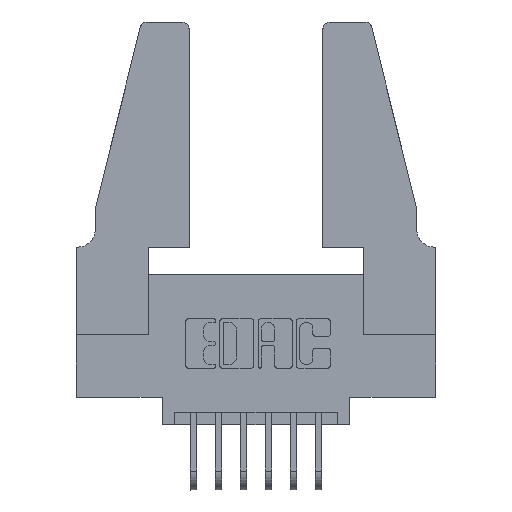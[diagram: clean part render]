
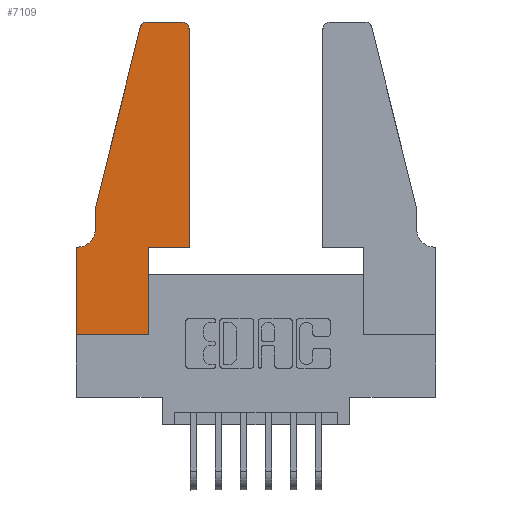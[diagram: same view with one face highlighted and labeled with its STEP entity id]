
A CAD part, top view. The second image highlights one B-rep face of the part: STEP entity #7109.
In plain terms, the highlighted planar face has unit normal (0, 0, 1).
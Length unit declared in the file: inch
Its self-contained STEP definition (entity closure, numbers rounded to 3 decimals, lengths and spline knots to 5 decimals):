
#90 = VECTOR ( 'NONE', #6976, 39.37008 ) ;
#445 = CARTESIAN_POINT ( 'NONE',  ( 0.25487, 1.22718, 0.37 ) ) ;
#467 = CIRCLE ( 'NONE', #1013, 0.03 ) ;
#564 = LINE ( 'NONE', #9493, #90 ) ;
#575 = PLANE ( 'NONE',  #3090 ) ;
#854 = CARTESIAN_POINT ( 'NONE',  ( 0.2605, 1.25, 0.37 ) ) ;
#901 = CIRCLE ( 'NONE', #8744, 0.03 ) ;
#1013 = AXIS2_PLACEMENT_3D ( 'NONE', #11137, #6403, #11711 ) ;
#1124 = CARTESIAN_POINT ( 'NONE',  ( 0.0055, 0.35, 0.37 ) ) ;
#1144 = VECTOR ( 'NONE', #3939, 39.37008 ) ;
#1252 = DIRECTION ( 'NONE',  ( 1., 0., 0. ) ) ;
#1342 = VERTEX_POINT ( 'NONE', #8738 ) ;
#1375 = LINE ( 'NONE', #10201, #1144 ) ;
#1415 = CARTESIAN_POINT ( 'NONE',  ( 0.0755, 0.5, 0.37 ) ) ;
#1596 = CARTESIAN_POINT ( 'NONE',  ( 0.4505, 0.35, 0.37 ) ) ;
#1606 = CARTESIAN_POINT ( 'NONE',  ( 0.4505, 0.35, 0.37 ) ) ;
#1700 = VECTOR ( 'NONE', #6832, 39.37008 ) ;
#1903 = LINE ( 'NONE', #1606, #1700 ) ;
#2016 = CIRCLE ( 'NONE', #2622, 0.07 ) ;
#2067 = EDGE_CURVE ( 'NONE', #8220, #10209, #5675, .T. ) ;
#2543 = VERTEX_POINT ( 'NONE', #445 ) ;
#2622 = AXIS2_PLACEMENT_3D ( 'NONE', #9012, #3261, #9797 ) ;
#3036 = VERTEX_POINT ( 'NONE', #10850 ) ;
#3090 = AXIS2_PLACEMENT_3D ( 'NONE', #6055, #11513, #7043 ) ;
#3141 = DIRECTION ( 'NONE',  ( -1., 0., 0. ) ) ;
#3221 = EDGE_CURVE ( 'NONE', #1342, #3036, #5656, .T. ) ;
#3261 = DIRECTION ( 'NONE',  ( 0., 0., -1. ) ) ;
#3382 = VERTEX_POINT ( 'NONE', #11277 ) ;
#3421 = VECTOR ( 'NONE', #10020, 39.37008 ) ;
#3434 = LINE ( 'NONE', #9252, #3421 ) ;
#3480 = EDGE_CURVE ( 'NONE', #3382, #8220, #1903, .T. ) ;
#3519 = EDGE_CURVE ( 'NONE', #4197, #8986, #1375, .T. ) ;
#3616 = ORIENTED_EDGE ( 'NONE', *, *, #3221, .T. ) ;
#3647 = ORIENTED_EDGE ( 'NONE', *, *, #9417, .T. ) ;
#3939 = DIRECTION ( 'NONE',  ( -1., 0., 0. ) ) ;
#4197 = VERTEX_POINT ( 'NONE', #1124 ) ;
#4227 = VERTEX_POINT ( 'NONE', #6589 ) ;
#4261 = EDGE_CURVE ( 'NONE', #2543, #8161, #10535, .T. ) ;
#4739 = VECTOR ( 'NONE', #3141, 39.37008 ) ;
#4779 = DIRECTION ( 'NONE',  ( -0.239, -0.971, 0. ) ) ;
#5116 = DIRECTION ( 'NONE',  ( 0., 0., 1. ) ) ;
#5293 = DIRECTION ( 'NONE',  ( 0., -1., 0. ) ) ;
#5432 = EDGE_LOOP ( 'NONE', ( #3616, #3647, #5825, #6375, #6441, #7413, #7513, #7723, #8041, #8762, #8914, #9424 ) ) ;
#5610 = VECTOR ( 'NONE', #9142, 39.37008 ) ;
#5656 = LINE ( 'NONE', #854, #4739 ) ;
#5675 = LINE ( 'NONE', #9864, #5610 ) ;
#5825 = ORIENTED_EDGE ( 'NONE', *, *, #4261, .T. ) ;
#6029 = VERTEX_POINT ( 'NONE', #8243 ) ;
#6055 = CARTESIAN_POINT ( 'NONE',  ( 0., 0.35, 0.37 ) ) ;
#6306 = FACE_OUTER_BOUND ( 'NONE', #5432, .T. ) ;
#6375 = ORIENTED_EDGE ( 'NONE', *, *, #10624, .T. ) ;
#6403 = DIRECTION ( 'NONE',  ( 0., 0., 1. ) ) ;
#6441 = ORIENTED_EDGE ( 'NONE', *, *, #8485, .T. ) ;
#6589 = CARTESIAN_POINT ( 'NONE',  ( 0.2865, 0., 0.37 ) ) ;
#6744 = CARTESIAN_POINT ( 'NONE',  ( 0.4505, 1.22, 0.37 ) ) ;
#6767 = EDGE_CURVE ( 'NONE', #6029, #4227, #10068, .T. ) ;
#6832 = DIRECTION ( 'NONE',  ( 1., 0., 0. ) ) ;
#6976 = DIRECTION ( 'NONE',  ( 0., -1., 0. ) ) ;
#7043 = DIRECTION ( 'NONE',  ( 1., 0., 0. ) ) ;
#7109 = ADVANCED_FACE ( 'NONE', ( #6306 ), #575, .T. ) ;
#7413 = ORIENTED_EDGE ( 'NONE', *, *, #3519, .T. ) ;
#7513 = ORIENTED_EDGE ( 'NONE', *, *, #11350, .T. ) ;
#7723 = ORIENTED_EDGE ( 'NONE', *, *, #6767, .T. ) ;
#7967 = CARTESIAN_POINT ( 'NONE',  ( 0., 0.35, 0.37 ) ) ;
#8041 = ORIENTED_EDGE ( 'NONE', *, *, #8070, .T. ) ;
#8070 = EDGE_CURVE ( 'NONE', #4227, #3382, #3434, .T. ) ;
#8161 = VERTEX_POINT ( 'NONE', #10781 ) ;
#8220 = VERTEX_POINT ( 'NONE', #1596 ) ;
#8243 = CARTESIAN_POINT ( 'NONE',  ( 0., 0., 0.37 ) ) ;
#8485 = EDGE_CURVE ( 'NONE', #9573, #4197, #2016, .T. ) ;
#8738 = CARTESIAN_POINT ( 'NONE',  ( 0.4205, 1.25, 0.37 ) ) ;
#8744 = AXIS2_PLACEMENT_3D ( 'NONE', #10275, #5116, #10927 ) ;
#8762 = ORIENTED_EDGE ( 'NONE', *, *, #3480, .T. ) ;
#8852 = EDGE_CURVE ( 'NONE', #10209, #1342, #901, .T. ) ;
#8914 = ORIENTED_EDGE ( 'NONE', *, *, #2067, .T. ) ;
#8986 = VERTEX_POINT ( 'NONE', #7967 ) ;
#9012 = CARTESIAN_POINT ( 'NONE',  ( 0.0055, 0.42, 0.37 ) ) ;
#9142 = DIRECTION ( 'NONE',  ( 0., 1., 0. ) ) ;
#9252 = CARTESIAN_POINT ( 'NONE',  ( 0.2865, 0.35, 0.37 ) ) ;
#9417 = EDGE_CURVE ( 'NONE', #3036, #2543, #467, .T. ) ;
#9424 = ORIENTED_EDGE ( 'NONE', *, *, #8852, .T. ) ;
#9493 = CARTESIAN_POINT ( 'NONE',  ( 0.0755, 0.5, 0.37 ) ) ;
#9504 = VECTOR ( 'NONE', #5293, 39.37008 ) ;
#9548 = LINE ( 'NONE', #10397, #9504 ) ;
#9573 = VERTEX_POINT ( 'NONE', #10548 ) ;
#9797 = DIRECTION ( 'NONE',  ( -1., 0., 0. ) ) ;
#9864 = CARTESIAN_POINT ( 'NONE',  ( 0.4505, 0.35, 0.37 ) ) ;
#10020 = DIRECTION ( 'NONE',  ( 0., 1., 0. ) ) ;
#10040 = VECTOR ( 'NONE', #1252, 39.37008 ) ;
#10068 = LINE ( 'NONE', #11232, #10040 ) ;
#10201 = CARTESIAN_POINT ( 'NONE',  ( 0.0755, 0.35, 0.37 ) ) ;
#10209 = VERTEX_POINT ( 'NONE', #6744 ) ;
#10275 = CARTESIAN_POINT ( 'NONE',  ( 0.4205, 1.22, 0.37 ) ) ;
#10397 = CARTESIAN_POINT ( 'NONE',  ( 0., 0., 0.37 ) ) ;
#10535 = LINE ( 'NONE', #1415, #10576 ) ;
#10548 = CARTESIAN_POINT ( 'NONE',  ( 0.0755, 0.42, 0.37 ) ) ;
#10576 = VECTOR ( 'NONE', #4779, 39.37008 ) ;
#10624 = EDGE_CURVE ( 'NONE', #8161, #9573, #564, .T. ) ;
#10781 = CARTESIAN_POINT ( 'NONE',  ( 0.0755, 0.5, 0.37 ) ) ;
#10850 = CARTESIAN_POINT ( 'NONE',  ( 0.284, 1.25, 0.37 ) ) ;
#10927 = DIRECTION ( 'NONE',  ( 1., 0., 0. ) ) ;
#11137 = CARTESIAN_POINT ( 'NONE',  ( 0.284, 1.22, 0.37 ) ) ;
#11232 = CARTESIAN_POINT ( 'NONE',  ( 0., 0., 0.37 ) ) ;
#11277 = CARTESIAN_POINT ( 'NONE',  ( 0.2865, 0.35, 0.37 ) ) ;
#11350 = EDGE_CURVE ( 'NONE', #8986, #6029, #9548, .T. ) ;
#11513 = DIRECTION ( 'NONE',  ( 0., 0., 1. ) ) ;
#11711 = DIRECTION ( 'NONE',  ( 1., 0., 0. ) ) ;
